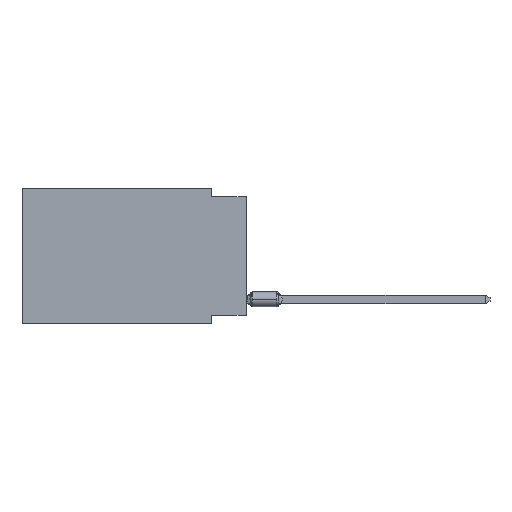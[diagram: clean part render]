
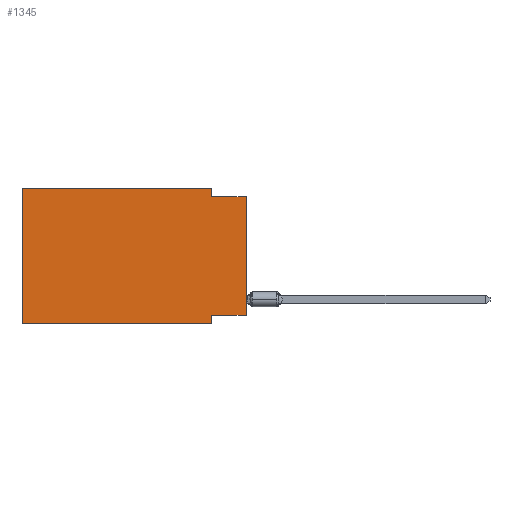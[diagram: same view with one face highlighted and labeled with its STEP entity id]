
A CAD part, left-side view. The second image highlights one B-rep face of the part: STEP entity #1345.
In plain terms, the highlighted planar face has unit normal (-1, 0, 0).
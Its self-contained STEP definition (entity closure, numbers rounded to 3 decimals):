
#441 = CARTESIAN_POINT ( 'NONE',  ( 0., 16.383, 0. ) ) ;
#696 = VERTEX_POINT ( 'NONE', #18842 ) ;
#868 = EDGE_CURVE ( 'NONE', #696, #8788, #4631, .T. ) ;
#1345 = ADVANCED_FACE ( 'NONE', ( #3124 ), #7874, .F. ) ;
#1381 = LINE ( 'NONE', #4547, #15481 ) ;
#1482 = CARTESIAN_POINT ( 'NONE',  ( 0., 16.383, 0. ) ) ;
#1544 = CARTESIAN_POINT ( 'NONE',  ( 0., 16.383, 0. ) ) ;
#1617 = CARTESIAN_POINT ( 'NONE',  ( 0., 16.383, -9.906 ) ) ;
#2354 = ORIENTED_EDGE ( 'NONE', *, *, #4555, .T. ) ;
#2507 = VECTOR ( 'NONE', #8530, 1000. ) ;
#2682 = LINE ( 'NONE', #1482, #5913 ) ;
#3124 = FACE_OUTER_BOUND ( 'NONE', #12951, .T. ) ;
#3347 = CARTESIAN_POINT ( 'NONE',  ( 0., 0., -0.635 ) ) ;
#3785 = VERTEX_POINT ( 'NONE', #3347 ) ;
#3946 = ORIENTED_EDGE ( 'NONE', *, *, #14951, .F. ) ;
#4023 = VECTOR ( 'NONE', #5322, 1000. ) ;
#4160 = CARTESIAN_POINT ( 'NONE',  ( 0., 2.54, -9.906 ) ) ;
#4163 = LINE ( 'NONE', #17864, #2507 ) ;
#4547 = CARTESIAN_POINT ( 'NONE',  ( 0., 0., -9.271 ) ) ;
#4555 = EDGE_CURVE ( 'NONE', #696, #6355, #7459, .T. ) ;
#4631 = LINE ( 'NONE', #441, #17814 ) ;
#5152 = AXIS2_PLACEMENT_3D ( 'NONE', #15219, #13634, #7759 ) ;
#5263 = VECTOR ( 'NONE', #9915, 1000. ) ;
#5322 = DIRECTION ( 'NONE',  ( 0., -1., 0. ) ) ;
#5546 = VECTOR ( 'NONE', #13717, 1000. ) ;
#5562 = ORIENTED_EDGE ( 'NONE', *, *, #11086, .F. ) ;
#5750 = DIRECTION ( 'NONE',  ( 0., -1., 0. ) ) ;
#5757 = ORIENTED_EDGE ( 'NONE', *, *, #7391, .F. ) ;
#5870 = VERTEX_POINT ( 'NONE', #17101 ) ;
#5913 = VECTOR ( 'NONE', #5750, 1000. ) ;
#6355 = VERTEX_POINT ( 'NONE', #9832 ) ;
#6401 = CARTESIAN_POINT ( 'NONE',  ( 0., 2.54, -9.271 ) ) ;
#6527 = EDGE_CURVE ( 'NONE', #19016, #18082, #1381, .T. ) ;
#6542 = EDGE_CURVE ( 'NONE', #19016, #3785, #17867, .T. ) ;
#7391 = EDGE_CURVE ( 'NONE', #18082, #6355, #14579, .T. ) ;
#7459 = LINE ( 'NONE', #1617, #5546 ) ;
#7759 = DIRECTION ( 'NONE',  ( 0., 0., -1. ) ) ;
#7874 = PLANE ( 'NONE',  #5152 ) ;
#8047 = CARTESIAN_POINT ( 'NONE',  ( 0., 2.54, -0.635 ) ) ;
#8530 = DIRECTION ( 'NONE',  ( 0., 0., -1. ) ) ;
#8788 = VERTEX_POINT ( 'NONE', #1544 ) ;
#9660 = ORIENTED_EDGE ( 'NONE', *, *, #6542, .T. ) ;
#9751 = CARTESIAN_POINT ( 'NONE',  ( 0., 0., -9.271 ) ) ;
#9832 = CARTESIAN_POINT ( 'NONE',  ( 0., 2.54, -9.906 ) ) ;
#9915 = DIRECTION ( 'NONE',  ( 0., 0., -1. ) ) ;
#10472 = ORIENTED_EDGE ( 'NONE', *, *, #868, .F. ) ;
#10599 = DIRECTION ( 'NONE',  ( 0., 1., 0. ) ) ;
#11086 = EDGE_CURVE ( 'NONE', #5870, #17484, #4163, .T. ) ;
#11982 = VECTOR ( 'NONE', #14879, 1000. ) ;
#12843 = LINE ( 'NONE', #18930, #4023 ) ;
#12951 = EDGE_LOOP ( 'NONE', ( #9660, #3946, #5562, #16542, #10472, #2354, #5757, #13288 ) ) ;
#13288 = ORIENTED_EDGE ( 'NONE', *, *, #6527, .F. ) ;
#13634 = DIRECTION ( 'NONE',  ( 1., 0., 0. ) ) ;
#13717 = DIRECTION ( 'NONE',  ( 0., -1., 0. ) ) ;
#14579 = LINE ( 'NONE', #4160, #5263 ) ;
#14879 = DIRECTION ( 'NONE',  ( 0., 0., 1. ) ) ;
#14951 = EDGE_CURVE ( 'NONE', #17484, #3785, #12843, .T. ) ;
#15219 = CARTESIAN_POINT ( 'NONE',  ( 0., 16.383, 0. ) ) ;
#15334 = DIRECTION ( 'NONE',  ( 0., 0., 1. ) ) ;
#15481 = VECTOR ( 'NONE', #10599, 1000. ) ;
#16369 = CARTESIAN_POINT ( 'NONE',  ( 0., 0., 0. ) ) ;
#16388 = EDGE_CURVE ( 'NONE', #8788, #5870, #2682, .T. ) ;
#16542 = ORIENTED_EDGE ( 'NONE', *, *, #16388, .F. ) ;
#17101 = CARTESIAN_POINT ( 'NONE',  ( 0., 2.54, 0. ) ) ;
#17484 = VERTEX_POINT ( 'NONE', #8047 ) ;
#17814 = VECTOR ( 'NONE', #15334, 1000. ) ;
#17864 = CARTESIAN_POINT ( 'NONE',  ( 0., 2.54, 0. ) ) ;
#17867 = LINE ( 'NONE', #16369, #11982 ) ;
#18082 = VERTEX_POINT ( 'NONE', #6401 ) ;
#18842 = CARTESIAN_POINT ( 'NONE',  ( 0., 16.383, -9.906 ) ) ;
#18930 = CARTESIAN_POINT ( 'NONE',  ( 0., 0., -0.635 ) ) ;
#19016 = VERTEX_POINT ( 'NONE', #9751 ) ;
